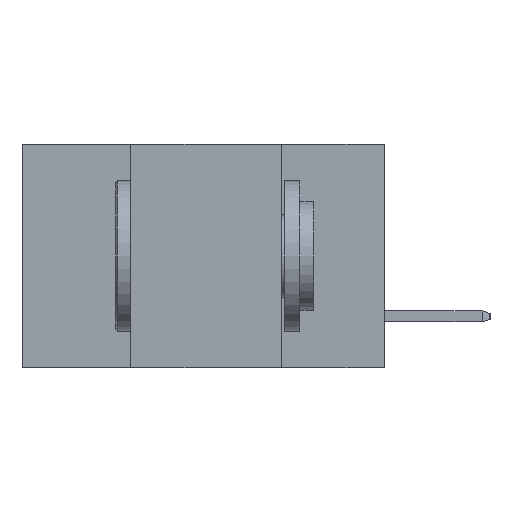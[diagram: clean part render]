
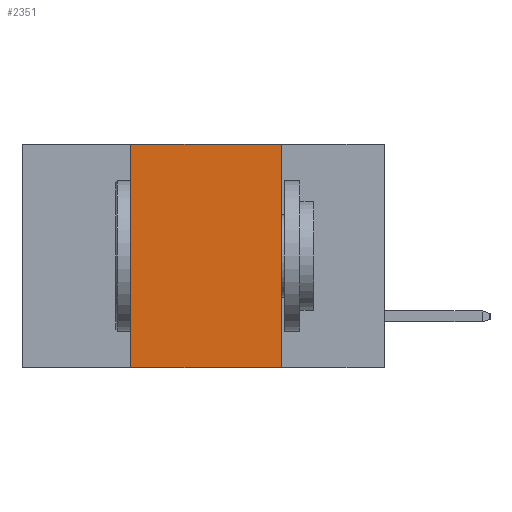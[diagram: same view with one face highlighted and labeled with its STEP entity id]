
A CAD part, left-side view. The second image highlights one B-rep face of the part: STEP entity #2351.
In plain terms, the highlighted planar face has unit normal (-1, 0, 0).
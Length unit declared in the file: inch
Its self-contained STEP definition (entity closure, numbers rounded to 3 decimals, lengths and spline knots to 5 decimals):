
#351 = VECTOR ( 'NONE', #3307, 39.37008 ) ;
#658 = FACE_OUTER_BOUND ( 'NONE', #14121, .T. ) ;
#692 = EDGE_CURVE ( 'NONE', #15416, #6314, #7772, .T. ) ;
#1119 = VECTOR ( 'NONE', #2100, 39.37008 ) ;
#1317 = CARTESIAN_POINT ( 'NONE',  ( 0., 0.6, 0. ) ) ;
#1680 = CARTESIAN_POINT ( 'NONE',  ( 0., 0.6, -0.37 ) ) ;
#2100 = DIRECTION ( 'NONE',  ( 0., -1., 0. ) ) ;
#2329 = LINE ( 'NONE', #19930, #6589 ) ;
#2351 = ADVANCED_FACE ( 'NONE', ( #658 ), #19954, .F. ) ;
#3159 = DIRECTION ( 'NONE',  ( 0., 0., -1. ) ) ;
#3307 = DIRECTION ( 'NONE',  ( 0., -1., 0. ) ) ;
#4382 = ORIENTED_EDGE ( 'NONE', *, *, #20089, .F. ) ;
#4656 = LINE ( 'NONE', #1680, #351 ) ;
#4883 = VERTEX_POINT ( 'NONE', #12282 ) ;
#6314 = VERTEX_POINT ( 'NONE', #8259 ) ;
#6589 = VECTOR ( 'NONE', #10564, 39.37008 ) ;
#7270 = VECTOR ( 'NONE', #8006, 39.37008 ) ;
#7714 = DIRECTION ( 'NONE',  ( 1., 0., 0. ) ) ;
#7772 = LINE ( 'NONE', #7965, #7270 ) ;
#7875 = CARTESIAN_POINT ( 'NONE',  ( 0., 0.17, 0. ) ) ;
#7965 = CARTESIAN_POINT ( 'NONE',  ( 0., 0.17, 0. ) ) ;
#8006 = DIRECTION ( 'NONE',  ( 0., 0., -1. ) ) ;
#8259 = CARTESIAN_POINT ( 'NONE',  ( 0., 0.17, -0.37 ) ) ;
#8591 = ORIENTED_EDGE ( 'NONE', *, *, #19054, .T. ) ;
#9392 = AXIS2_PLACEMENT_3D ( 'NONE', #1317, #7714, #3159 ) ;
#9985 = CARTESIAN_POINT ( 'NONE',  ( 0., 0.6, 0. ) ) ;
#10564 = DIRECTION ( 'NONE',  ( 0., 0., 1. ) ) ;
#12039 = CARTESIAN_POINT ( 'NONE',  ( 0., 0.42, 0. ) ) ;
#12254 = ORIENTED_EDGE ( 'NONE', *, *, #692, .F. ) ;
#12282 = CARTESIAN_POINT ( 'NONE',  ( 0., 0.42, -0.37 ) ) ;
#13742 = LINE ( 'NONE', #9985, #1119 ) ;
#14121 = EDGE_LOOP ( 'NONE', ( #12254, #16440, #4382, #8591 ) ) ;
#15416 = VERTEX_POINT ( 'NONE', #7875 ) ;
#16440 = ORIENTED_EDGE ( 'NONE', *, *, #19215, .F. ) ;
#16522 = VERTEX_POINT ( 'NONE', #12039 ) ;
#19054 = EDGE_CURVE ( 'NONE', #4883, #6314, #4656, .T. ) ;
#19215 = EDGE_CURVE ( 'NONE', #16522, #15416, #13742, .T. ) ;
#19930 = CARTESIAN_POINT ( 'NONE',  ( 0., 0.42, 0. ) ) ;
#19954 = PLANE ( 'NONE',  #9392 ) ;
#20089 = EDGE_CURVE ( 'NONE', #4883, #16522, #2329, .T. ) ;
